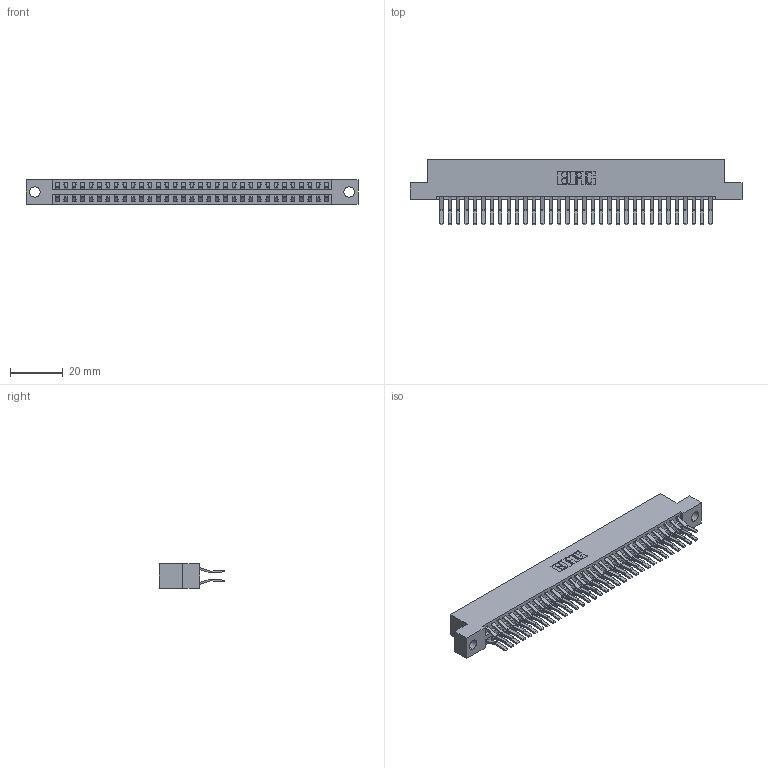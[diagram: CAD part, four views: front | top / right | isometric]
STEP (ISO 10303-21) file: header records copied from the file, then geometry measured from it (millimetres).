
FILE_DESCRIPTION (( 'STEP AP203' ), '1' );
FILE_NAME ('396-066-560-204.STEP', '2018-09-08T20:25:51', ( '' ), ( '' ), 'SwSTEP 2.0', 'SolidWorks 2016', '' );
FILE_SCHEMA (( 'CONFIG_CONTROL_DESIGN' ));
Length unit declared in the file: inch
Products named in the file (3): 346 Part_Flush Mounting Lugs - 0.156 Dia-TH; 345-292-001_560 Tail; 396-066-560-204
Assembly tree (67 placements, depth 2):
  396-066-560-204
    346 Part_Flush Mounting Lugs - 0.156 Dia-TH
    345-292-001_560 Tail  x66
Bounding box: 125.35 x 24.78 x 9.4 mm (x, y, z)
Volume: 12497.9 mm3; surface area: 18005.3 mm2
Topology: 67 solids, 67 shells, 3686 faces, 10955 edges, 7214 vertices
Faces by surface type: plane 2386, cylinder 1300
Entity records: 22839 total; most frequent: CARTESIAN_POINT 3776, ORIENTED_EDGE 3710, DIRECTION 3383, EDGE_CURVE 1855, LINE 1587, VECTOR 1587, VERTEX_POINT 1234, AXIS2_PLACEMENT_3D 898
